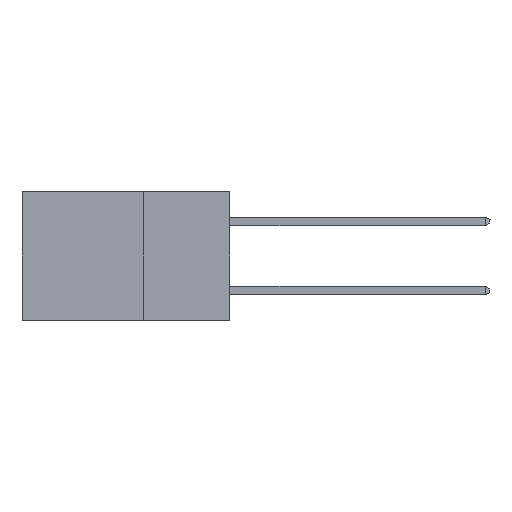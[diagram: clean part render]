
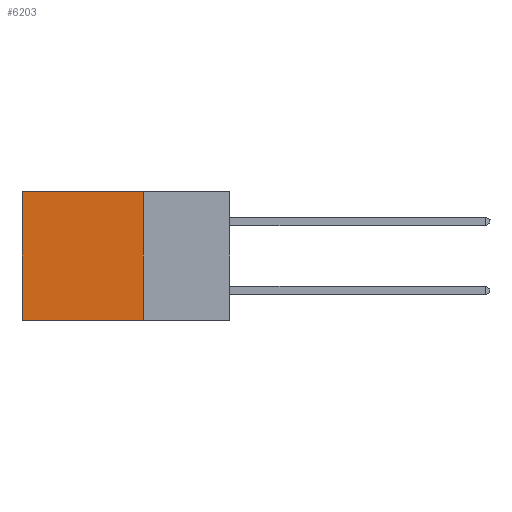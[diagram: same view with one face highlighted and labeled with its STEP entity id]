
A CAD part, left-side view. The second image highlights one B-rep face of the part: STEP entity #6203.
In plain terms, the highlighted planar face has unit normal (-1, 0, 0).
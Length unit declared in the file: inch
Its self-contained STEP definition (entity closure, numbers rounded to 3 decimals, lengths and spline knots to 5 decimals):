
#319 = LINE ( 'NONE', #15756, #10696 ) ;
#409 = VERTEX_POINT ( 'NONE', #14901 ) ;
#836 = PLANE ( 'NONE',  #17420 ) ;
#1522 = VECTOR ( 'NONE', #8885, 39.37008 ) ;
#2674 = EDGE_CURVE ( 'NONE', #2830, #8898, #13162, .T. ) ;
#2830 = VERTEX_POINT ( 'NONE', #5385 ) ;
#3044 = DIRECTION ( 'NONE',  ( 0., 0., -1. ) ) ;
#5385 = CARTESIAN_POINT ( 'NONE',  ( 0.298, 0.25, 0. ) ) ;
#5612 = DIRECTION ( 'NONE',  ( 0., 0., -1. ) ) ;
#5673 = VERTEX_POINT ( 'NONE', #21916 ) ;
#6128 = ORIENTED_EDGE ( 'NONE', *, *, #13556, .F. ) ;
#6203 = ADVANCED_FACE ( 'NONE', ( #11064 ), #836, .F. ) ;
#6348 = LINE ( 'NONE', #22297, #15897 ) ;
#6891 = CARTESIAN_POINT ( 'NONE',  ( 0.298, 0.25, -0.37 ) ) ;
#8399 = VECTOR ( 'NONE', #22491, 39.37008 ) ;
#8885 = DIRECTION ( 'NONE',  ( 0., 1., 0. ) ) ;
#8898 = VERTEX_POINT ( 'NONE', #10267 ) ;
#9100 = CARTESIAN_POINT ( 'NONE',  ( 0.298, 0.25, 0. ) ) ;
#10267 = CARTESIAN_POINT ( 'NONE',  ( 0.298, 0.6, 0. ) ) ;
#10696 = VECTOR ( 'NONE', #5612, 39.37008 ) ;
#11064 = FACE_OUTER_BOUND ( 'NONE', #19950, .T. ) ;
#13162 = LINE ( 'NONE', #24179, #8399 ) ;
#13556 = EDGE_CURVE ( 'NONE', #2830, #5673, #319, .T. ) ;
#14477 = ORIENTED_EDGE ( 'NONE', *, *, #26394, .F. ) ;
#14901 = CARTESIAN_POINT ( 'NONE',  ( 0.298, 0.6, -0.37 ) ) ;
#15274 = DIRECTION ( 'NONE',  ( 1., 0., 0. ) ) ;
#15756 = CARTESIAN_POINT ( 'NONE',  ( 0.298, 0.25, 0. ) ) ;
#15897 = VECTOR ( 'NONE', #18294, 39.37008 ) ;
#17420 = AXIS2_PLACEMENT_3D ( 'NONE', #9100, #15274, #3044 ) ;
#17943 = LINE ( 'NONE', #6891, #1522 ) ;
#18294 = DIRECTION ( 'NONE',  ( 0., 0., -1. ) ) ;
#18903 = EDGE_CURVE ( 'NONE', #8898, #409, #6348, .T. ) ;
#19950 = EDGE_LOOP ( 'NONE', ( #24310, #14477, #6128, #20364 ) ) ;
#20364 = ORIENTED_EDGE ( 'NONE', *, *, #2674, .T. ) ;
#21916 = CARTESIAN_POINT ( 'NONE',  ( 0.298, 0.25, -0.37 ) ) ;
#22297 = CARTESIAN_POINT ( 'NONE',  ( 0.298, 0.6, 0. ) ) ;
#22491 = DIRECTION ( 'NONE',  ( 0., 1., 0. ) ) ;
#24179 = CARTESIAN_POINT ( 'NONE',  ( 0.298, 0.25, 0. ) ) ;
#24310 = ORIENTED_EDGE ( 'NONE', *, *, #18903, .T. ) ;
#26394 = EDGE_CURVE ( 'NONE', #5673, #409, #17943, .T. ) ;
